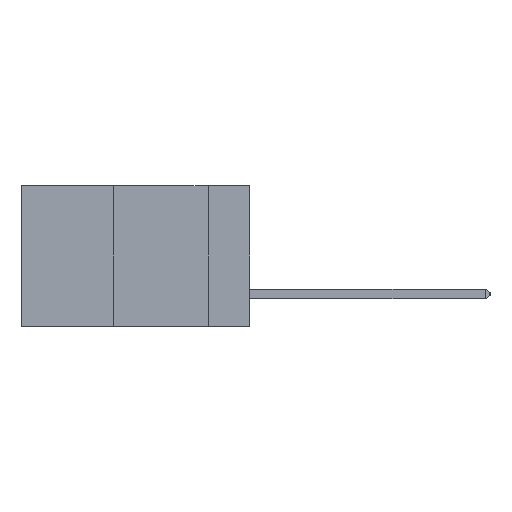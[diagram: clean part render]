
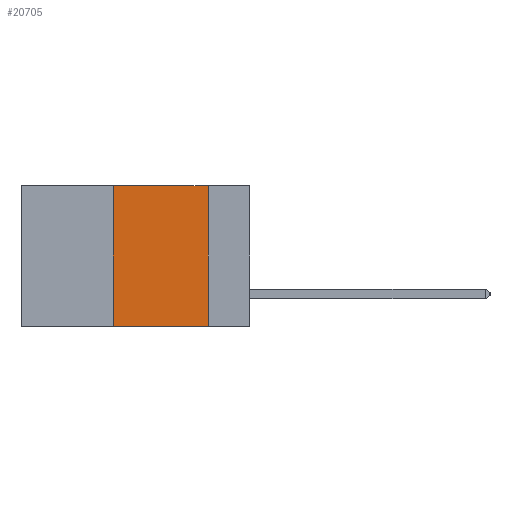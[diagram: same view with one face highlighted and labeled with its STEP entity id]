
A CAD part, left-side view. The second image highlights one B-rep face of the part: STEP entity #20705.
In plain terms, the highlighted planar face has unit normal (-1, 0, 0).
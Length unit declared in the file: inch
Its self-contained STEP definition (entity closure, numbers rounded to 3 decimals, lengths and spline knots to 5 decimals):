
#70 = LINE ( 'NONE', #6772, #8760 ) ;
#739 = CARTESIAN_POINT ( 'NONE',  ( 0., 0.6, 0. ) ) ;
#804 = DIRECTION ( 'NONE',  ( 0., 0., -1. ) ) ;
#1788 = EDGE_CURVE ( 'NONE', #7971, #15957, #15775, .T. ) ;
#2753 = CARTESIAN_POINT ( 'NONE',  ( 0., 0.36, 0. ) ) ;
#3193 = VECTOR ( 'NONE', #15572, 39.37008 ) ;
#5462 = ORIENTED_EDGE ( 'NONE', *, *, #7117, .F. ) ;
#5475 = DIRECTION ( 'NONE',  ( 0., -1., 0. ) ) ;
#6772 = CARTESIAN_POINT ( 'NONE',  ( 0., 0.36, 0. ) ) ;
#7075 = CARTESIAN_POINT ( 'NONE',  ( 0., 0.11, -0.37 ) ) ;
#7117 = EDGE_CURVE ( 'NONE', #13218, #13662, #18012, .T. ) ;
#7178 = EDGE_LOOP ( 'NONE', ( #17724, #5462, #16426, #10661 ) ) ;
#7971 = VERTEX_POINT ( 'NONE', #9197 ) ;
#8760 = VECTOR ( 'NONE', #18278, 39.37008 ) ;
#9197 = CARTESIAN_POINT ( 'NONE',  ( 0., 0.36, -0.37 ) ) ;
#9872 = AXIS2_PLACEMENT_3D ( 'NONE', #739, #10631, #804 ) ;
#9902 = LINE ( 'NONE', #15165, #20947 ) ;
#10631 = DIRECTION ( 'NONE',  ( 1., 0., 0. ) ) ;
#10661 = ORIENTED_EDGE ( 'NONE', *, *, #1788, .T. ) ;
#13218 = VERTEX_POINT ( 'NONE', #2753 ) ;
#13638 = VECTOR ( 'NONE', #5475, 39.37008 ) ;
#13662 = VERTEX_POINT ( 'NONE', #18797 ) ;
#13679 = CARTESIAN_POINT ( 'NONE',  ( 0., 0.6, 0. ) ) ;
#14000 = FACE_OUTER_BOUND ( 'NONE', #7178, .T. ) ;
#15165 = CARTESIAN_POINT ( 'NONE',  ( 0., 0.11, 0. ) ) ;
#15572 = DIRECTION ( 'NONE',  ( 0., -1., 0. ) ) ;
#15775 = LINE ( 'NONE', #20532, #3193 ) ;
#15957 = VERTEX_POINT ( 'NONE', #7075 ) ;
#16331 = EDGE_CURVE ( 'NONE', #7971, #13218, #70, .T. ) ;
#16426 = ORIENTED_EDGE ( 'NONE', *, *, #16331, .F. ) ;
#16799 = DIRECTION ( 'NONE',  ( 0., 0., -1. ) ) ;
#17724 = ORIENTED_EDGE ( 'NONE', *, *, #20569, .F. ) ;
#18012 = LINE ( 'NONE', #13679, #13638 ) ;
#18278 = DIRECTION ( 'NONE',  ( 0., 0., 1. ) ) ;
#18797 = CARTESIAN_POINT ( 'NONE',  ( 0., 0.11, 0. ) ) ;
#20473 = PLANE ( 'NONE',  #9872 ) ;
#20532 = CARTESIAN_POINT ( 'NONE',  ( 0., 0.6, -0.37 ) ) ;
#20569 = EDGE_CURVE ( 'NONE', #13662, #15957, #9902, .T. ) ;
#20705 = ADVANCED_FACE ( 'NONE', ( #14000 ), #20473, .F. ) ;
#20947 = VECTOR ( 'NONE', #16799, 39.37008 ) ;
